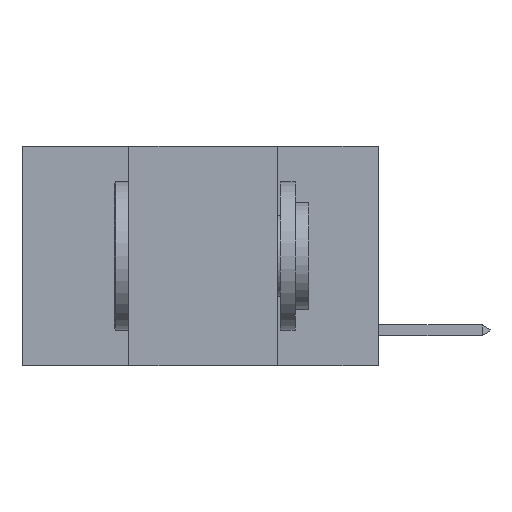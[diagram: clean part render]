
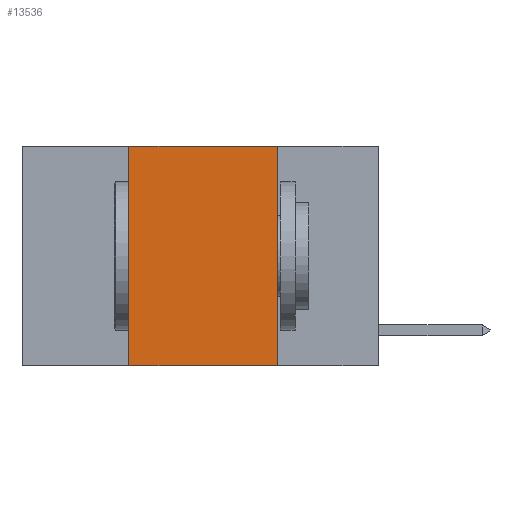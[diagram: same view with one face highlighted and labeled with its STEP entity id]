
A CAD part, left-side view. The second image highlights one B-rep face of the part: STEP entity #13536.
In plain terms, the highlighted planar face has unit normal (-1, 0, 0).
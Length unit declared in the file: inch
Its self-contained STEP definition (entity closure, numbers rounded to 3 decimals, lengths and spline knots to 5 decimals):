
#183 = VERTEX_POINT ( 'NONE', #681 ) ;
#191 = CARTESIAN_POINT ( 'NONE',  ( 0., 0.6, -0.37 ) ) ;
#206 = CARTESIAN_POINT ( 'NONE',  ( 0., 0.17, 0. ) ) ;
#429 = CARTESIAN_POINT ( 'NONE',  ( 0., 0.42, 0. ) ) ;
#681 = CARTESIAN_POINT ( 'NONE',  ( 0., 0.42, -0.37 ) ) ;
#1053 = VECTOR ( 'NONE', #1080, 39.37008 ) ;
#1080 = DIRECTION ( 'NONE',  ( 0., -1., 0. ) ) ;
#2119 = CARTESIAN_POINT ( 'NONE',  ( 0., 0.6, 0. ) ) ;
#2425 = VERTEX_POINT ( 'NONE', #7464 ) ;
#2604 = DIRECTION ( 'NONE',  ( 0., 0., 1. ) ) ;
#2611 = EDGE_CURVE ( 'NONE', #2425, #10708, #7232, .T. ) ;
#3232 = LINE ( 'NONE', #2119, #1053 ) ;
#3698 = LINE ( 'NONE', #429, #8852 ) ;
#3718 = CARTESIAN_POINT ( 'NONE',  ( 0., 0.17, -0.37 ) ) ;
#4784 = DIRECTION ( 'NONE',  ( 0., 0., -1. ) ) ;
#5295 = EDGE_CURVE ( 'NONE', #183, #5730, #3698, .T. ) ;
#5340 = CARTESIAN_POINT ( 'NONE',  ( 0., 0.6, 0. ) ) ;
#5723 = DIRECTION ( 'NONE',  ( 0., -1., 0. ) ) ;
#5730 = VERTEX_POINT ( 'NONE', #13095 ) ;
#5857 = EDGE_CURVE ( 'NONE', #5730, #2425, #3232, .T. ) ;
#5887 = EDGE_LOOP ( 'NONE', ( #6365, #13071, #12521, #8946 ) ) ;
#6365 = ORIENTED_EDGE ( 'NONE', *, *, #2611, .F. ) ;
#6426 = EDGE_CURVE ( 'NONE', #183, #10708, #12577, .T. ) ;
#6476 = VECTOR ( 'NONE', #5723, 39.37008 ) ;
#7232 = LINE ( 'NONE', #206, #11587 ) ;
#7464 = CARTESIAN_POINT ( 'NONE',  ( 0., 0.17, 0. ) ) ;
#7804 = DIRECTION ( 'NONE',  ( 0., 0., -1. ) ) ;
#8852 = VECTOR ( 'NONE', #2604, 39.37008 ) ;
#8938 = PLANE ( 'NONE',  #9484 ) ;
#8946 = ORIENTED_EDGE ( 'NONE', *, *, #6426, .T. ) ;
#9484 = AXIS2_PLACEMENT_3D ( 'NONE', #5340, #12475, #7804 ) ;
#10708 = VERTEX_POINT ( 'NONE', #3718 ) ;
#11587 = VECTOR ( 'NONE', #4784, 39.37008 ) ;
#12234 = FACE_OUTER_BOUND ( 'NONE', #5887, .T. ) ;
#12475 = DIRECTION ( 'NONE',  ( 1., 0., 0. ) ) ;
#12521 = ORIENTED_EDGE ( 'NONE', *, *, #5295, .F. ) ;
#12577 = LINE ( 'NONE', #191, #6476 ) ;
#13071 = ORIENTED_EDGE ( 'NONE', *, *, #5857, .F. ) ;
#13095 = CARTESIAN_POINT ( 'NONE',  ( 0., 0.42, 0. ) ) ;
#13536 = ADVANCED_FACE ( 'NONE', ( #12234 ), #8938, .F. ) ;
